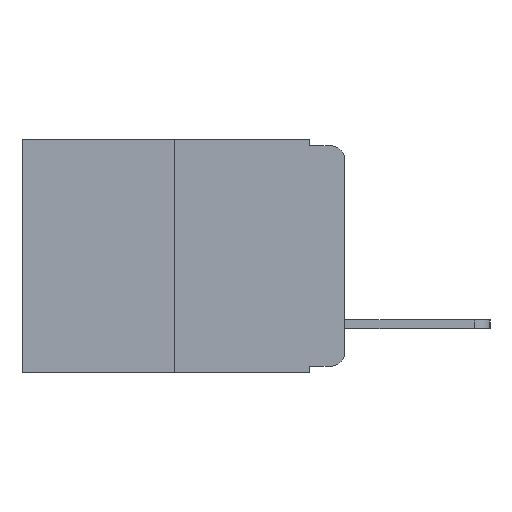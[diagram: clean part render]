
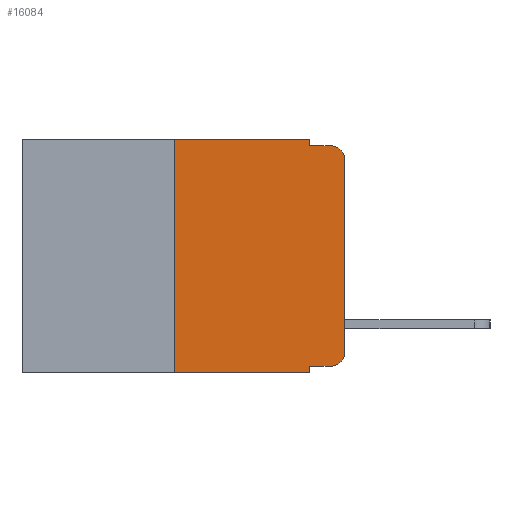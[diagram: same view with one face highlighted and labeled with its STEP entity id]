
A CAD part, left-side view. The second image highlights one B-rep face of the part: STEP entity #16084.
In plain terms, the highlighted planar face has unit normal (-1, 0, 0).
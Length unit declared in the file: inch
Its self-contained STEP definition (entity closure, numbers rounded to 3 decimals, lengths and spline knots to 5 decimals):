
#220 = CARTESIAN_POINT ( 'NONE',  ( 0., 0.051, 0. ) ) ;
#345 = EDGE_CURVE ( 'NONE', #2459, #4366, #6058, .T. ) ;
#865 = FACE_OUTER_BOUND ( 'NONE', #3164, .T. ) ;
#1021 = ORIENTED_EDGE ( 'NONE', *, *, #345, .F. ) ;
#1074 = EDGE_CURVE ( 'NONE', #5002, #4366, #12996, .T. ) ;
#1211 = DIRECTION ( 'NONE',  ( 0., 0., -1. ) ) ;
#1227 = DIRECTION ( 'NONE',  ( -1., 0., 0. ) ) ;
#1373 = VERTEX_POINT ( 'NONE', #12707 ) ;
#1482 = CARTESIAN_POINT ( 'NONE',  ( 0., 0.051, -0.01 ) ) ;
#1686 = ORIENTED_EDGE ( 'NONE', *, *, #14932, .T. ) ;
#2185 = VECTOR ( 'NONE', #12155, 39.37008 ) ;
#2459 = VERTEX_POINT ( 'NONE', #1482 ) ;
#2591 = ORIENTED_EDGE ( 'NONE', *, *, #7280, .T. ) ;
#2900 = VECTOR ( 'NONE', #6711, 39.37008 ) ;
#2936 = CARTESIAN_POINT ( 'NONE',  ( 0., 0.051, -0.343 ) ) ;
#2985 = CARTESIAN_POINT ( 'NONE',  ( 0., 0.051, -0.01 ) ) ;
#3127 = CIRCLE ( 'NONE', #5261, 0.02 ) ;
#3164 = EDGE_LOOP ( 'NONE', ( #2591, #7832, #1021, #4866, #5774, #10519, #15622, #4642, #16066, #1686 ) ) ;
#3909 = DIRECTION ( 'NONE',  ( 0., 0., -1. ) ) ;
#4366 = VERTEX_POINT ( 'NONE', #15615 ) ;
#4642 = ORIENTED_EDGE ( 'NONE', *, *, #7198, .F. ) ;
#4866 = ORIENTED_EDGE ( 'NONE', *, *, #6116, .F. ) ;
#4933 = CARTESIAN_POINT ( 'NONE',  ( 0., 0.473, 0. ) ) ;
#5002 = VERTEX_POINT ( 'NONE', #17035 ) ;
#5261 = AXIS2_PLACEMENT_3D ( 'NONE', #16814, #8310, #18216 ) ;
#5650 = CARTESIAN_POINT ( 'NONE',  ( 0., 0., -0.313 ) ) ;
#5774 = ORIENTED_EDGE ( 'NONE', *, *, #9060, .F. ) ;
#5789 = LINE ( 'NONE', #13959, #18059 ) ;
#6015 = AXIS2_PLACEMENT_3D ( 'NONE', #4933, #16384, #7876 ) ;
#6058 = LINE ( 'NONE', #2985, #2185 ) ;
#6116 = EDGE_CURVE ( 'NONE', #12559, #2459, #5789, .T. ) ;
#6335 = CARTESIAN_POINT ( 'NONE',  ( 0., 0.25, 0. ) ) ;
#6711 = DIRECTION ( 'NONE',  ( 0., -1., 0. ) ) ;
#7044 = VERTEX_POINT ( 'NONE', #5650 ) ;
#7142 = VERTEX_POINT ( 'NONE', #2936 ) ;
#7198 = EDGE_CURVE ( 'NONE', #18529, #7142, #10067, .T. ) ;
#7280 = EDGE_CURVE ( 'NONE', #7044, #5002, #15831, .T. ) ;
#7446 = DIRECTION ( 'NONE',  ( 0., 0., -1. ) ) ;
#7448 = EDGE_CURVE ( 'NONE', #18251, #17601, #9812, .T. ) ;
#7791 = DIRECTION ( 'NONE',  ( 0., 0., 1. ) ) ;
#7832 = ORIENTED_EDGE ( 'NONE', *, *, #1074, .T. ) ;
#7876 = DIRECTION ( 'NONE',  ( 0., 0., -1. ) ) ;
#7993 = EDGE_CURVE ( 'NONE', #18251, #7142, #17538, .T. ) ;
#8310 = DIRECTION ( 'NONE',  ( -1., 0., 0. ) ) ;
#9060 = EDGE_CURVE ( 'NONE', #17601, #12559, #11106, .T. ) ;
#9424 = AXIS2_PLACEMENT_3D ( 'NONE', #12581, #1227, #1211 ) ;
#9812 = LINE ( 'NONE', #6335, #16908 ) ;
#10067 = LINE ( 'NONE', #220, #13861 ) ;
#10122 = DIRECTION ( 'NONE',  ( 0., -1., 0. ) ) ;
#10158 = DIRECTION ( 'NONE',  ( 0., 0., 1. ) ) ;
#10484 = CARTESIAN_POINT ( 'NONE',  ( 0., 0.25, -0.343 ) ) ;
#10519 = ORIENTED_EDGE ( 'NONE', *, *, #7448, .F. ) ;
#10563 = DIRECTION ( 'NONE',  ( 0., -1., 0. ) ) ;
#11106 = LINE ( 'NONE', #16548, #18163 ) ;
#12099 = VECTOR ( 'NONE', #10158, 39.37008 ) ;
#12155 = DIRECTION ( 'NONE',  ( 0., -1., 0. ) ) ;
#12559 = VERTEX_POINT ( 'NONE', #18329 ) ;
#12581 = CARTESIAN_POINT ( 'NONE',  ( 0., 0.02, -0.03 ) ) ;
#12707 = CARTESIAN_POINT ( 'NONE',  ( 0., 0.02, -0.333 ) ) ;
#12996 = CIRCLE ( 'NONE', #9424, 0.02 ) ;
#13004 = CARTESIAN_POINT ( 'NONE',  ( 0., 0.25, 0. ) ) ;
#13539 = PLANE ( 'NONE',  #6015 ) ;
#13775 = VECTOR ( 'NONE', #10563, 39.37008 ) ;
#13861 = VECTOR ( 'NONE', #3909, 39.37008 ) ;
#13940 = LINE ( 'NONE', #15216, #2900 ) ;
#13959 = CARTESIAN_POINT ( 'NONE',  ( 0., 0.051, 0. ) ) ;
#14932 = EDGE_CURVE ( 'NONE', #1373, #7044, #3127, .T. ) ;
#15216 = CARTESIAN_POINT ( 'NONE',  ( 0., 0.051, -0.333 ) ) ;
#15615 = CARTESIAN_POINT ( 'NONE',  ( 0., 0.02, -0.01 ) ) ;
#15622 = ORIENTED_EDGE ( 'NONE', *, *, #7993, .T. ) ;
#15673 = EDGE_CURVE ( 'NONE', #18529, #1373, #13940, .T. ) ;
#15831 = LINE ( 'NONE', #16556, #12099 ) ;
#16066 = ORIENTED_EDGE ( 'NONE', *, *, #15673, .T. ) ;
#16084 = ADVANCED_FACE ( 'NONE', ( #865 ), #13539, .F. ) ;
#16204 = CARTESIAN_POINT ( 'NONE',  ( 0., 0.473, -0.343 ) ) ;
#16384 = DIRECTION ( 'NONE',  ( 1., 0., 0. ) ) ;
#16548 = CARTESIAN_POINT ( 'NONE',  ( 0., 0.473, 0. ) ) ;
#16556 = CARTESIAN_POINT ( 'NONE',  ( 0., 0., 0. ) ) ;
#16751 = CARTESIAN_POINT ( 'NONE',  ( 0., 0.051, -0.333 ) ) ;
#16814 = CARTESIAN_POINT ( 'NONE',  ( 0., 0.02, -0.313 ) ) ;
#16908 = VECTOR ( 'NONE', #7791, 39.37008 ) ;
#17035 = CARTESIAN_POINT ( 'NONE',  ( 0., 0., -0.03 ) ) ;
#17538 = LINE ( 'NONE', #16204, #13775 ) ;
#17601 = VERTEX_POINT ( 'NONE', #13004 ) ;
#18059 = VECTOR ( 'NONE', #7446, 39.37008 ) ;
#18163 = VECTOR ( 'NONE', #10122, 39.37008 ) ;
#18216 = DIRECTION ( 'NONE',  ( 0., 0., -1. ) ) ;
#18251 = VERTEX_POINT ( 'NONE', #10484 ) ;
#18329 = CARTESIAN_POINT ( 'NONE',  ( 0., 0.051, 0. ) ) ;
#18529 = VERTEX_POINT ( 'NONE', #16751 ) ;
